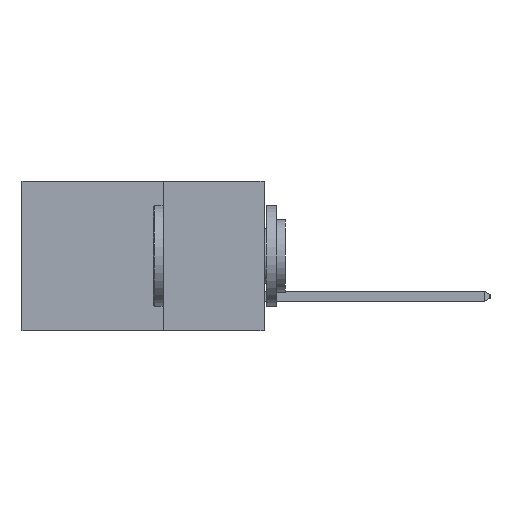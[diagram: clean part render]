
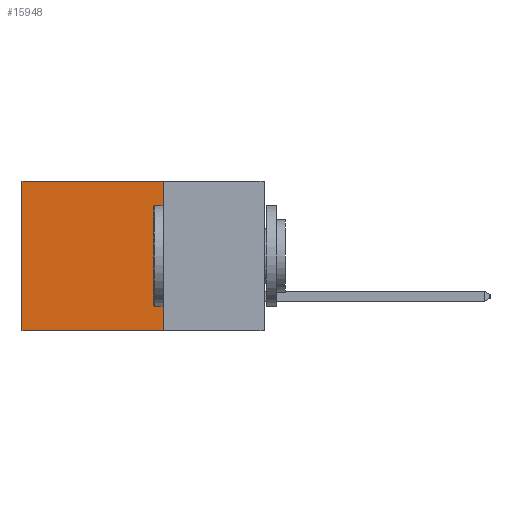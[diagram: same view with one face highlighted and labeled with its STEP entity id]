
A CAD part, left-side view. The second image highlights one B-rep face of the part: STEP entity #15948.
In plain terms, the highlighted planar face has unit normal (-1, 0, 0).
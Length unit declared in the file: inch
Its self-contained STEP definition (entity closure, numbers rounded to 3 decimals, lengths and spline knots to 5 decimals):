
#472 = VERTEX_POINT ( 'NONE', #3376 ) ;
#1927 = VECTOR ( 'NONE', #16283, 39.37008 ) ;
#2411 = LINE ( 'NONE', #12450, #14811 ) ;
#2806 = DIRECTION ( 'NONE',  ( 0., 1., 0. ) ) ;
#3376 = CARTESIAN_POINT ( 'NONE',  ( 0.298, 0.6, 0. ) ) ;
#3716 = CARTESIAN_POINT ( 'NONE',  ( 0.298, 0.25, 0. ) ) ;
#4122 = AXIS2_PLACEMENT_3D ( 'NONE', #8446, #10930, #28165 ) ;
#5960 = PLANE ( 'NONE',  #4122 ) ;
#8446 = CARTESIAN_POINT ( 'NONE',  ( 0.298, 0.25, 0. ) ) ;
#8490 = EDGE_CURVE ( 'NONE', #22452, #15260, #21941, .T. ) ;
#8687 = DIRECTION ( 'NONE',  ( 0., 0., -1. ) ) ;
#10645 = ORIENTED_EDGE ( 'NONE', *, *, #8490, .F. ) ;
#10930 = DIRECTION ( 'NONE',  ( 1., 0., 0. ) ) ;
#11260 = EDGE_CURVE ( 'NONE', #472, #15260, #2411, .T. ) ;
#11380 = EDGE_LOOP ( 'NONE', ( #22166, #10645, #18145, #20713 ) ) ;
#11525 = FACE_OUTER_BOUND ( 'NONE', #11380, .T. ) ;
#12293 = EDGE_CURVE ( 'NONE', #26749, #472, #22447, .T. ) ;
#12450 = CARTESIAN_POINT ( 'NONE',  ( 0.298, 0.6, 0. ) ) ;
#14620 = VECTOR ( 'NONE', #2806, 39.37008 ) ;
#14811 = VECTOR ( 'NONE', #27201, 39.37008 ) ;
#15260 = VERTEX_POINT ( 'NONE', #23182 ) ;
#15350 = EDGE_CURVE ( 'NONE', #26749, #22452, #20107, .T. ) ;
#15382 = CARTESIAN_POINT ( 'NONE',  ( 0.298, 0.25, -0.37 ) ) ;
#15948 = ADVANCED_FACE ( 'NONE', ( #11525 ), #5960, .F. ) ;
#16283 = DIRECTION ( 'NONE',  ( 0., 1., 0. ) ) ;
#18145 = ORIENTED_EDGE ( 'NONE', *, *, #15350, .F. ) ;
#20107 = LINE ( 'NONE', #3716, #23543 ) ;
#20124 = CARTESIAN_POINT ( 'NONE',  ( 0.298, 0.25, -0.37 ) ) ;
#20713 = ORIENTED_EDGE ( 'NONE', *, *, #12293, .T. ) ;
#20748 = CARTESIAN_POINT ( 'NONE',  ( 0.298, 0.25, 0. ) ) ;
#21941 = LINE ( 'NONE', #20124, #14620 ) ;
#22166 = ORIENTED_EDGE ( 'NONE', *, *, #11260, .T. ) ;
#22447 = LINE ( 'NONE', #31049, #1927 ) ;
#22452 = VERTEX_POINT ( 'NONE', #15382 ) ;
#23182 = CARTESIAN_POINT ( 'NONE',  ( 0.298, 0.6, -0.37 ) ) ;
#23543 = VECTOR ( 'NONE', #8687, 39.37008 ) ;
#26749 = VERTEX_POINT ( 'NONE', #20748 ) ;
#27201 = DIRECTION ( 'NONE',  ( 0., 0., -1. ) ) ;
#28165 = DIRECTION ( 'NONE',  ( 0., 0., -1. ) ) ;
#31049 = CARTESIAN_POINT ( 'NONE',  ( 0.298, 0.25, 0. ) ) ;
